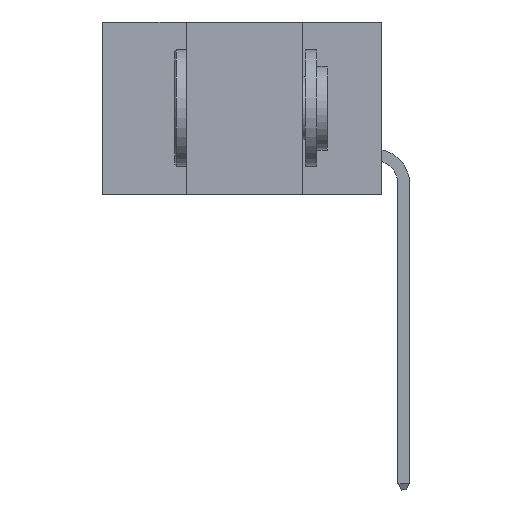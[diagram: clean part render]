
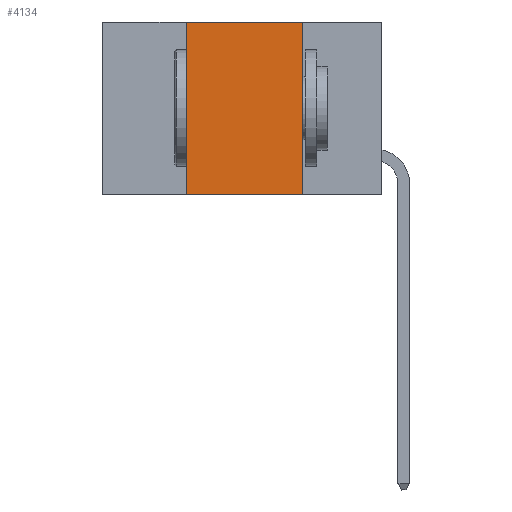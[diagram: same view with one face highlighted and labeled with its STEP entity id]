
A CAD part, left-side view. The second image highlights one B-rep face of the part: STEP entity #4134.
In plain terms, the highlighted planar face has unit normal (-1, 0, 0).
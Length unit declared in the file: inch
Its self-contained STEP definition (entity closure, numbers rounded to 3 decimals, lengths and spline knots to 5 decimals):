
#40 = EDGE_CURVE ( 'NONE', #8592, #13222, #12677, .T. ) ;
#978 = ORIENTED_EDGE ( 'NONE', *, *, #19771, .F. ) ;
#1462 = CARTESIAN_POINT ( 'NONE',  ( 0., 0.6, 0. ) ) ;
#1542 = ORIENTED_EDGE ( 'NONE', *, *, #15135, .F. ) ;
#1850 = CARTESIAN_POINT ( 'NONE',  ( 0., 0.6, 0. ) ) ;
#2222 = AXIS2_PLACEMENT_3D ( 'NONE', #1850, #14074, #15814 ) ;
#2886 = EDGE_LOOP ( 'NONE', ( #1542, #978, #14885, #3090 ) ) ;
#2912 = VECTOR ( 'NONE', #18751, 39.37008 ) ;
#3090 = ORIENTED_EDGE ( 'NONE', *, *, #16102, .T. ) ;
#3312 = CARTESIAN_POINT ( 'NONE',  ( 0., 0.42, 0. ) ) ;
#3995 = LINE ( 'NONE', #6541, #2912 ) ;
#4134 = ADVANCED_FACE ( 'NONE', ( #8099 ), #12223, .F. ) ;
#6149 = CARTESIAN_POINT ( 'NONE',  ( 0., 0.17, -0.37 ) ) ;
#6541 = CARTESIAN_POINT ( 'NONE',  ( 0., 0.17, 0. ) ) ;
#6993 = LINE ( 'NONE', #12325, #12451 ) ;
#7655 = VECTOR ( 'NONE', #18999, 39.37008 ) ;
#8099 = FACE_OUTER_BOUND ( 'NONE', #2886, .T. ) ;
#8592 = VERTEX_POINT ( 'NONE', #9371 ) ;
#9371 = CARTESIAN_POINT ( 'NONE',  ( 0., 0.42, -0.37 ) ) ;
#11062 = CARTESIAN_POINT ( 'NONE',  ( 0., 0.42, 0. ) ) ;
#11864 = VERTEX_POINT ( 'NONE', #15141 ) ;
#12223 = PLANE ( 'NONE',  #2222 ) ;
#12296 = VERTEX_POINT ( 'NONE', #6149 ) ;
#12325 = CARTESIAN_POINT ( 'NONE',  ( 0., 0.6, -0.37 ) ) ;
#12451 = VECTOR ( 'NONE', #14388, 39.37008 ) ;
#12677 = LINE ( 'NONE', #11062, #21092 ) ;
#13222 = VERTEX_POINT ( 'NONE', #3312 ) ;
#14074 = DIRECTION ( 'NONE',  ( 1., 0., 0. ) ) ;
#14388 = DIRECTION ( 'NONE',  ( 0., -1., 0. ) ) ;
#14583 = DIRECTION ( 'NONE',  ( 0., 0., 1. ) ) ;
#14885 = ORIENTED_EDGE ( 'NONE', *, *, #40, .F. ) ;
#15135 = EDGE_CURVE ( 'NONE', #11864, #12296, #3995, .T. ) ;
#15141 = CARTESIAN_POINT ( 'NONE',  ( 0., 0.17, 0. ) ) ;
#15814 = DIRECTION ( 'NONE',  ( 0., 0., -1. ) ) ;
#16102 = EDGE_CURVE ( 'NONE', #8592, #12296, #6993, .T. ) ;
#18751 = DIRECTION ( 'NONE',  ( 0., 0., -1. ) ) ;
#18999 = DIRECTION ( 'NONE',  ( 0., -1., 0. ) ) ;
#19771 = EDGE_CURVE ( 'NONE', #13222, #11864, #21556, .T. ) ;
#21092 = VECTOR ( 'NONE', #14583, 39.37008 ) ;
#21556 = LINE ( 'NONE', #1462, #7655 ) ;
